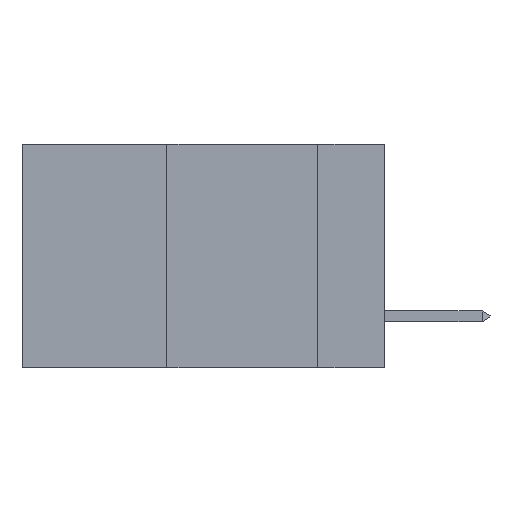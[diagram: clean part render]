
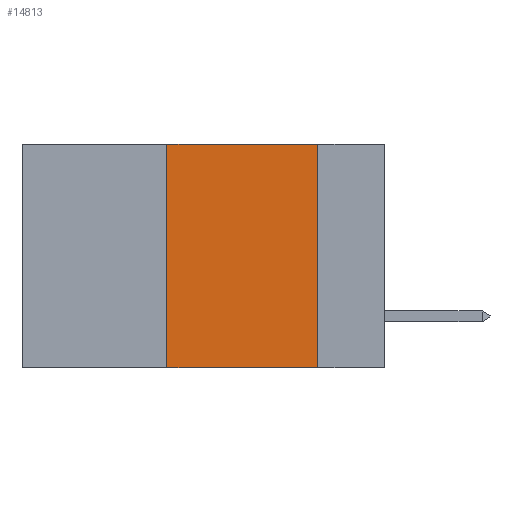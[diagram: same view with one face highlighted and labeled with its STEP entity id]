
A CAD part, left-side view. The second image highlights one B-rep face of the part: STEP entity #14813.
In plain terms, the highlighted planar face has unit normal (-1, 0, 0).
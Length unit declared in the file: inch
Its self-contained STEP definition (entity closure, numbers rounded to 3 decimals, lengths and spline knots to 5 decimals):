
#118 = LINE ( 'NONE', #14864, #15512 ) ;
#167 = ORIENTED_EDGE ( 'NONE', *, *, #15041, .T. ) ;
#349 = CARTESIAN_POINT ( 'NONE',  ( 0., 0.6, 0. ) ) ;
#895 = CARTESIAN_POINT ( 'NONE',  ( 0., 0.11, -0.37 ) ) ;
#1543 = ORIENTED_EDGE ( 'NONE', *, *, #20287, .F. ) ;
#1967 = LINE ( 'NONE', #19522, #6316 ) ;
#2030 = EDGE_CURVE ( 'NONE', #16307, #4198, #1967, .T. ) ;
#3588 = LINE ( 'NONE', #5346, #12728 ) ;
#3676 = CARTESIAN_POINT ( 'NONE',  ( 0., 0.36, 0. ) ) ;
#4198 = VERTEX_POINT ( 'NONE', #3676 ) ;
#5125 = DIRECTION ( 'NONE',  ( 0., -1., 0. ) ) ;
#5346 = CARTESIAN_POINT ( 'NONE',  ( 0., 0.6, -0.37 ) ) ;
#5782 = PLANE ( 'NONE',  #10066 ) ;
#6316 = VECTOR ( 'NONE', #14631, 39.37008 ) ;
#7215 = VECTOR ( 'NONE', #5125, 39.37008 ) ;
#7439 = CARTESIAN_POINT ( 'NONE',  ( 0., 0.6, 0. ) ) ;
#7921 = DIRECTION ( 'NONE',  ( 0., 0., -1. ) ) ;
#8424 = EDGE_CURVE ( 'NONE', #11894, #12184, #118, .T. ) ;
#8456 = DIRECTION ( 'NONE',  ( 0., -1., 0. ) ) ;
#8672 = CARTESIAN_POINT ( 'NONE',  ( 0., 0.36, -0.37 ) ) ;
#8751 = LINE ( 'NONE', #349, #7215 ) ;
#9094 = CARTESIAN_POINT ( 'NONE',  ( 0., 0.11, 0. ) ) ;
#9709 = ORIENTED_EDGE ( 'NONE', *, *, #8424, .F. ) ;
#10066 = AXIS2_PLACEMENT_3D ( 'NONE', #7439, #12115, #15340 ) ;
#11894 = VERTEX_POINT ( 'NONE', #9094 ) ;
#12115 = DIRECTION ( 'NONE',  ( 1., 0., 0. ) ) ;
#12184 = VERTEX_POINT ( 'NONE', #895 ) ;
#12728 = VECTOR ( 'NONE', #8456, 39.37008 ) ;
#13672 = FACE_OUTER_BOUND ( 'NONE', #18273, .T. ) ;
#14631 = DIRECTION ( 'NONE',  ( 0., 0., 1. ) ) ;
#14813 = ADVANCED_FACE ( 'NONE', ( #13672 ), #5782, .F. ) ;
#14864 = CARTESIAN_POINT ( 'NONE',  ( 0., 0.11, 0. ) ) ;
#15041 = EDGE_CURVE ( 'NONE', #16307, #12184, #3588, .T. ) ;
#15340 = DIRECTION ( 'NONE',  ( 0., 0., -1. ) ) ;
#15512 = VECTOR ( 'NONE', #7921, 39.37008 ) ;
#16307 = VERTEX_POINT ( 'NONE', #8672 ) ;
#18273 = EDGE_LOOP ( 'NONE', ( #9709, #1543, #19998, #167 ) ) ;
#19522 = CARTESIAN_POINT ( 'NONE',  ( 0., 0.36, 0. ) ) ;
#19998 = ORIENTED_EDGE ( 'NONE', *, *, #2030, .F. ) ;
#20287 = EDGE_CURVE ( 'NONE', #4198, #11894, #8751, .T. ) ;
